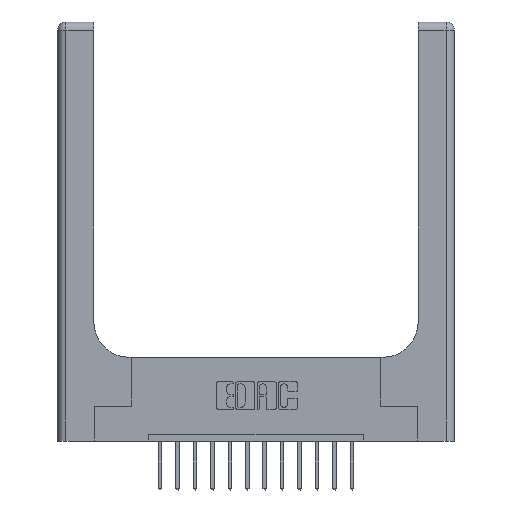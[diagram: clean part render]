
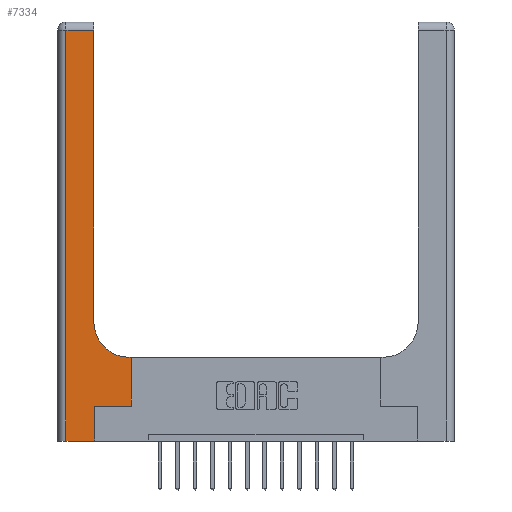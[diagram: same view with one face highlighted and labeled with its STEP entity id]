
A CAD part, top view. The second image highlights one B-rep face of the part: STEP entity #7334.
In plain terms, the highlighted planar face has unit normal (0, 0, 1).
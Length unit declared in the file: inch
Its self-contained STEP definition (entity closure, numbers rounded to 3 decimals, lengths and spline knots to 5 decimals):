
#36 = ORIENTED_EDGE ( 'NONE', *, *, #8018, .T. ) ;
#274 = CARTESIAN_POINT ( 'NONE',  ( 0., 0., 0.37 ) ) ;
#703 = ORIENTED_EDGE ( 'NONE', *, *, #11119, .T. ) ;
#706 = EDGE_CURVE ( 'NONE', #14797, #6703, #5201, .T. ) ;
#746 = EDGE_CURVE ( 'NONE', #9004, #4584, #2403, .T. ) ;
#755 = DIRECTION ( 'NONE',  ( 1., 0., 0. ) ) ;
#800 = ORIENTED_EDGE ( 'NONE', *, *, #706, .T. ) ;
#834 = VECTOR ( 'NONE', #13415, 39.37008 ) ;
#1443 = CARTESIAN_POINT ( 'NONE',  ( 0.528, 0.25, 0.37 ) ) ;
#1722 = DIRECTION ( 'NONE',  ( 0., 0., -1. ) ) ;
#2005 = CARTESIAN_POINT ( 'NONE',  ( 0.06, 2.94, 0.37 ) ) ;
#2165 = EDGE_CURVE ( 'NONE', #3545, #9004, #15673, .T. ) ;
#2403 = CIRCLE ( 'NONE', #15784, 0.25 ) ;
#2814 = VECTOR ( 'NONE', #5358, 39.37008 ) ;
#3340 = CARTESIAN_POINT ( 'NONE',  ( 0.06, 0., 0.37 ) ) ;
#3545 = VERTEX_POINT ( 'NONE', #12294 ) ;
#3917 = ORIENTED_EDGE ( 'NONE', *, *, #2165, .T. ) ;
#4319 = VECTOR ( 'NONE', #11074, 39.37008 ) ;
#4584 = VERTEX_POINT ( 'NONE', #10448 ) ;
#4868 = EDGE_LOOP ( 'NONE', ( #36, #16463, #12776, #800, #703, #5994, #10538, #3917, #9147 ) ) ;
#5157 = CARTESIAN_POINT ( 'NONE',  ( 0.265, 0.25, 0.37 ) ) ;
#5201 = LINE ( 'NONE', #274, #5784 ) ;
#5358 = DIRECTION ( 'NONE',  ( 1., 0., 0. ) ) ;
#5500 = CARTESIAN_POINT ( 'NONE',  ( 0.51, 0.6, 0.37 ) ) ;
#5629 = CARTESIAN_POINT ( 'NONE',  ( 0., 3., 0.37 ) ) ;
#5784 = VECTOR ( 'NONE', #7991, 39.37008 ) ;
#5994 = ORIENTED_EDGE ( 'NONE', *, *, #7913, .T. ) ;
#6703 = VERTEX_POINT ( 'NONE', #11416 ) ;
#6999 = LINE ( 'NONE', #8087, #10878 ) ;
#7095 = DIRECTION ( 'NONE',  ( -1., 0., 0. ) ) ;
#7135 = CARTESIAN_POINT ( 'NONE',  ( 0.265, 0., 0.37 ) ) ;
#7333 = CARTESIAN_POINT ( 'NONE',  ( 0.528, 0.25, 0.37 ) ) ;
#7334 = ADVANCED_FACE ( 'NONE', ( #7444 ), #13473, .F. ) ;
#7444 = FACE_OUTER_BOUND ( 'NONE', #4868, .T. ) ;
#7913 = EDGE_CURVE ( 'NONE', #11379, #15360, #16289, .T. ) ;
#7991 = DIRECTION ( 'NONE',  ( 1., 0., 0. ) ) ;
#8018 = EDGE_CURVE ( 'NONE', #4584, #10107, #6999, .T. ) ;
#8087 = CARTESIAN_POINT ( 'NONE',  ( 0.26, 3., 0.37 ) ) ;
#8214 = CARTESIAN_POINT ( 'NONE',  ( 0., 2.94, 0.37 ) ) ;
#8290 = DIRECTION ( 'NONE',  ( -1., 0., 0. ) ) ;
#8436 = DIRECTION ( 'NONE',  ( 0., 0., -1. ) ) ;
#8474 = DIRECTION ( 'NONE',  ( 0., -1., 0. ) ) ;
#8904 = VECTOR ( 'NONE', #11277, 39.37008 ) ;
#9004 = VERTEX_POINT ( 'NONE', #5500 ) ;
#9147 = ORIENTED_EDGE ( 'NONE', *, *, #746, .T. ) ;
#9407 = DIRECTION ( 'NONE',  ( 0., 1., 0. ) ) ;
#10107 = VERTEX_POINT ( 'NONE', #12823 ) ;
#10448 = CARTESIAN_POINT ( 'NONE',  ( 0.26, 0.85, 0.37 ) ) ;
#10538 = ORIENTED_EDGE ( 'NONE', *, *, #14928, .T. ) ;
#10878 = VECTOR ( 'NONE', #9407, 39.37008 ) ;
#11074 = DIRECTION ( 'NONE',  ( 0., 1., 0. ) ) ;
#11119 = EDGE_CURVE ( 'NONE', #6703, #11379, #12997, .T. ) ;
#11277 = DIRECTION ( 'NONE',  ( 0., 1., 0. ) ) ;
#11379 = VERTEX_POINT ( 'NONE', #5157 ) ;
#11416 = CARTESIAN_POINT ( 'NONE',  ( 0.265, 0., 0.37 ) ) ;
#12202 = VECTOR ( 'NONE', #8474, 39.37008 ) ;
#12294 = CARTESIAN_POINT ( 'NONE',  ( 0.528, 0.6, 0.37 ) ) ;
#12439 = CARTESIAN_POINT ( 'NONE',  ( 0.06, 3., 0.37 ) ) ;
#12776 = ORIENTED_EDGE ( 'NONE', *, *, #13239, .T. ) ;
#12823 = CARTESIAN_POINT ( 'NONE',  ( 0.26, 2.94, 0.37 ) ) ;
#12997 = LINE ( 'NONE', #7135, #4319 ) ;
#13239 = EDGE_CURVE ( 'NONE', #15646, #14797, #15424, .T. ) ;
#13256 = VECTOR ( 'NONE', #8290, 39.37008 ) ;
#13349 = LINE ( 'NONE', #7333, #8904 ) ;
#13415 = DIRECTION ( 'NONE',  ( -1., 0., 0. ) ) ;
#13473 = PLANE ( 'NONE',  #16593 ) ;
#14562 = LINE ( 'NONE', #8214, #834 ) ;
#14625 = CARTESIAN_POINT ( 'NONE',  ( 0.26, 0.6, 0.37 ) ) ;
#14797 = VERTEX_POINT ( 'NONE', #3340 ) ;
#14823 = EDGE_CURVE ( 'NONE', #10107, #15646, #14562, .T. ) ;
#14928 = EDGE_CURVE ( 'NONE', #15360, #3545, #13349, .T. ) ;
#15157 = CARTESIAN_POINT ( 'NONE',  ( 0.51, 0.85, 0.37 ) ) ;
#15360 = VERTEX_POINT ( 'NONE', #1443 ) ;
#15424 = LINE ( 'NONE', #12439, #12202 ) ;
#15646 = VERTEX_POINT ( 'NONE', #2005 ) ;
#15651 = CARTESIAN_POINT ( 'NONE',  ( 0.265, 0.25, 0.37 ) ) ;
#15673 = LINE ( 'NONE', #14625, #13256 ) ;
#15784 = AXIS2_PLACEMENT_3D ( 'NONE', #15157, #8436, #755 ) ;
#16289 = LINE ( 'NONE', #15651, #2814 ) ;
#16463 = ORIENTED_EDGE ( 'NONE', *, *, #14823, .T. ) ;
#16593 = AXIS2_PLACEMENT_3D ( 'NONE', #5629, #1722, #7095 ) ;
